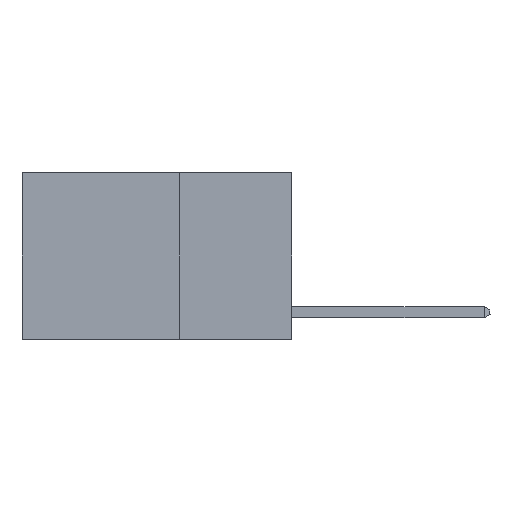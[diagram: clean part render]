
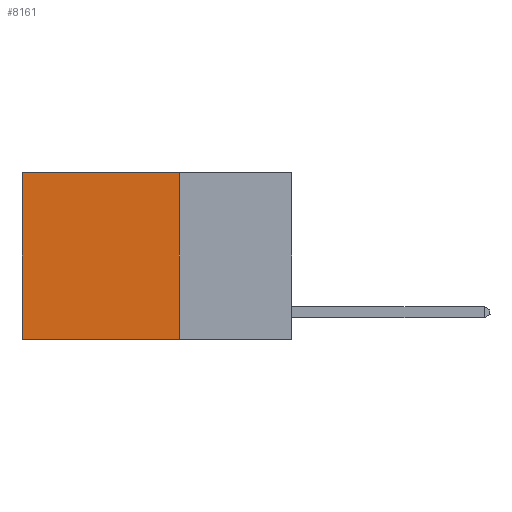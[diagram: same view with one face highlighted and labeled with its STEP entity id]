
A CAD part, left-side view. The second image highlights one B-rep face of the part: STEP entity #8161.
In plain terms, the highlighted planar face has unit normal (-1, 0, 0).
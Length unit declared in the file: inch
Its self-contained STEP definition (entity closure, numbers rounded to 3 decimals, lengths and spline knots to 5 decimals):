
#2099 = VECTOR ( 'NONE', #6520, 39.37008 ) ;
#2330 = EDGE_CURVE ( 'NONE', #21736, #15774, #10127, .T. ) ;
#2379 = ORIENTED_EDGE ( 'NONE', *, *, #8633, .T. ) ;
#3543 = VERTEX_POINT ( 'NONE', #6913 ) ;
#4340 = FACE_OUTER_BOUND ( 'NONE', #16368, .T. ) ;
#6520 = DIRECTION ( 'NONE',  ( 0., 0., -1. ) ) ;
#6913 = CARTESIAN_POINT ( 'NONE',  ( 0.2625, 0.25, -0.37 ) ) ;
#7174 = ORIENTED_EDGE ( 'NONE', *, *, #2330, .T. ) ;
#8161 = ADVANCED_FACE ( 'NONE', ( #4340 ), #17363, .F. ) ;
#8633 = EDGE_CURVE ( 'NONE', #15774, #10077, #18979, .T. ) ;
#10077 = VERTEX_POINT ( 'NONE', #18715 ) ;
#10127 = LINE ( 'NONE', #16803, #27010 ) ;
#10265 = DIRECTION ( 'NONE',  ( 0., 1., 0. ) ) ;
#10977 = DIRECTION ( 'NONE',  ( 0., 0., -1. ) ) ;
#11751 = EDGE_CURVE ( 'NONE', #3543, #10077, #16529, .T. ) ;
#12290 = CARTESIAN_POINT ( 'NONE',  ( 0.2625, 0.25, -0.37 ) ) ;
#14383 = EDGE_CURVE ( 'NONE', #21736, #3543, #20004, .T. ) ;
#15609 = AXIS2_PLACEMENT_3D ( 'NONE', #26029, #21761, #10977 ) ;
#15763 = CARTESIAN_POINT ( 'NONE',  ( 0.2625, 0.25, 0. ) ) ;
#15774 = VERTEX_POINT ( 'NONE', #18414 ) ;
#16189 = ORIENTED_EDGE ( 'NONE', *, *, #14383, .F. ) ;
#16368 = EDGE_LOOP ( 'NONE', ( #2379, #21113, #16189, #7174 ) ) ;
#16529 = LINE ( 'NONE', #12290, #27790 ) ;
#16803 = CARTESIAN_POINT ( 'NONE',  ( 0.2625, 0.25, 0. ) ) ;
#17363 = PLANE ( 'NONE',  #15609 ) ;
#18414 = CARTESIAN_POINT ( 'NONE',  ( 0.2625, 0.6, 0. ) ) ;
#18715 = CARTESIAN_POINT ( 'NONE',  ( 0.2625, 0.6, -0.37 ) ) ;
#18979 = LINE ( 'NONE', #19122, #2099 ) ;
#19122 = CARTESIAN_POINT ( 'NONE',  ( 0.2625, 0.6, 0. ) ) ;
#19603 = DIRECTION ( 'NONE',  ( 0., 0., -1. ) ) ;
#20004 = LINE ( 'NONE', #15763, #27211 ) ;
#21060 = DIRECTION ( 'NONE',  ( 0., 1., 0. ) ) ;
#21113 = ORIENTED_EDGE ( 'NONE', *, *, #11751, .F. ) ;
#21736 = VERTEX_POINT ( 'NONE', #26470 ) ;
#21761 = DIRECTION ( 'NONE',  ( 1., 0., 0. ) ) ;
#26029 = CARTESIAN_POINT ( 'NONE',  ( 0.2625, 0.25, 0. ) ) ;
#26470 = CARTESIAN_POINT ( 'NONE',  ( 0.2625, 0.25, 0. ) ) ;
#27010 = VECTOR ( 'NONE', #10265, 39.37008 ) ;
#27211 = VECTOR ( 'NONE', #19603, 39.37008 ) ;
#27790 = VECTOR ( 'NONE', #21060, 39.37008 ) ;
